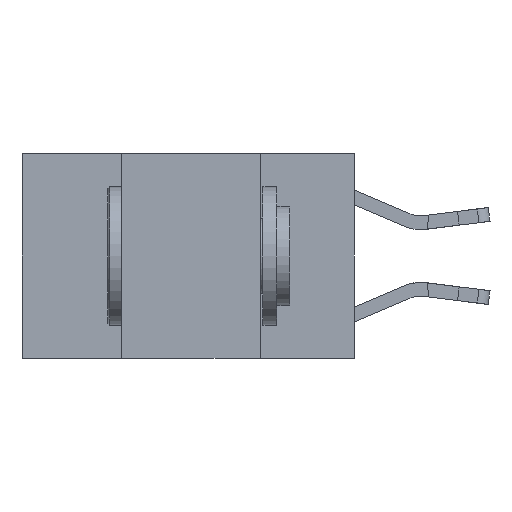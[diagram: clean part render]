
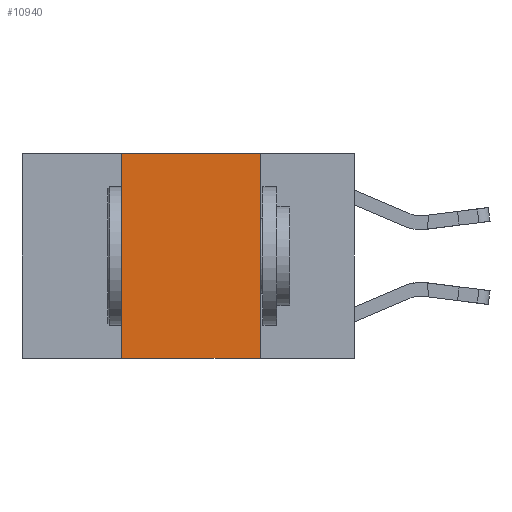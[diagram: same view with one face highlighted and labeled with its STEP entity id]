
A CAD part, left-side view. The second image highlights one B-rep face of the part: STEP entity #10940.
In plain terms, the highlighted planar face has unit normal (-1, 0, 0).
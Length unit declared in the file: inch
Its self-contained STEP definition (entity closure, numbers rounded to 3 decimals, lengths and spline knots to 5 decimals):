
#786 = LINE ( 'NONE', #9958, #13268 ) ;
#1318 = CARTESIAN_POINT ( 'NONE',  ( 0., 0.6, 0. ) ) ;
#1545 = AXIS2_PLACEMENT_3D ( 'NONE', #1318, #15695, #22879 ) ;
#2031 = CARTESIAN_POINT ( 'NONE',  ( 0., 0.17, 0. ) ) ;
#2639 = DIRECTION ( 'NONE',  ( 0., 0., 1. ) ) ;
#3084 = FACE_OUTER_BOUND ( 'NONE', #10850, .T. ) ;
#4265 = CARTESIAN_POINT ( 'NONE',  ( 0., 0.42, 0. ) ) ;
#4558 = CARTESIAN_POINT ( 'NONE',  ( 0., 0.42, -0.37 ) ) ;
#6257 = VERTEX_POINT ( 'NONE', #4265 ) ;
#7237 = VECTOR ( 'NONE', #2639, 39.37008 ) ;
#7316 = DIRECTION ( 'NONE',  ( 0., 0., -1. ) ) ;
#7365 = CARTESIAN_POINT ( 'NONE',  ( 0., 0.6, 0. ) ) ;
#7480 = DIRECTION ( 'NONE',  ( 0., -1., 0. ) ) ;
#7856 = ORIENTED_EDGE ( 'NONE', *, *, #12802, .T. ) ;
#7965 = DIRECTION ( 'NONE',  ( 0., -1., 0. ) ) ;
#8108 = VECTOR ( 'NONE', #7480, 39.37008 ) ;
#8200 = ORIENTED_EDGE ( 'NONE', *, *, #19782, .F. ) ;
#8745 = ORIENTED_EDGE ( 'NONE', *, *, #13890, .F. ) ;
#9818 = LINE ( 'NONE', #11494, #7237 ) ;
#9958 = CARTESIAN_POINT ( 'NONE',  ( 0., 0.6, -0.37 ) ) ;
#10265 = PLANE ( 'NONE',  #1545 ) ;
#10850 = EDGE_LOOP ( 'NONE', ( #8200, #19134, #8745, #7856 ) ) ;
#10940 = ADVANCED_FACE ( 'NONE', ( #3084 ), #10265, .F. ) ;
#11107 = LINE ( 'NONE', #2031, #21665 ) ;
#11494 = CARTESIAN_POINT ( 'NONE',  ( 0., 0.42, 0. ) ) ;
#12802 = EDGE_CURVE ( 'NONE', #19150, #16572, #786, .T. ) ;
#13268 = VECTOR ( 'NONE', #7965, 39.37008 ) ;
#13890 = EDGE_CURVE ( 'NONE', #19150, #6257, #9818, .T. ) ;
#15695 = DIRECTION ( 'NONE',  ( 1., 0., 0. ) ) ;
#15997 = VERTEX_POINT ( 'NONE', #16159 ) ;
#16159 = CARTESIAN_POINT ( 'NONE',  ( 0., 0.17, 0. ) ) ;
#16330 = LINE ( 'NONE', #7365, #8108 ) ;
#16572 = VERTEX_POINT ( 'NONE', #17898 ) ;
#17580 = EDGE_CURVE ( 'NONE', #6257, #15997, #16330, .T. ) ;
#17898 = CARTESIAN_POINT ( 'NONE',  ( 0., 0.17, -0.37 ) ) ;
#19134 = ORIENTED_EDGE ( 'NONE', *, *, #17580, .F. ) ;
#19150 = VERTEX_POINT ( 'NONE', #4558 ) ;
#19782 = EDGE_CURVE ( 'NONE', #15997, #16572, #11107, .T. ) ;
#21665 = VECTOR ( 'NONE', #7316, 39.37008 ) ;
#22879 = DIRECTION ( 'NONE',  ( 0., 0., -1. ) ) ;
